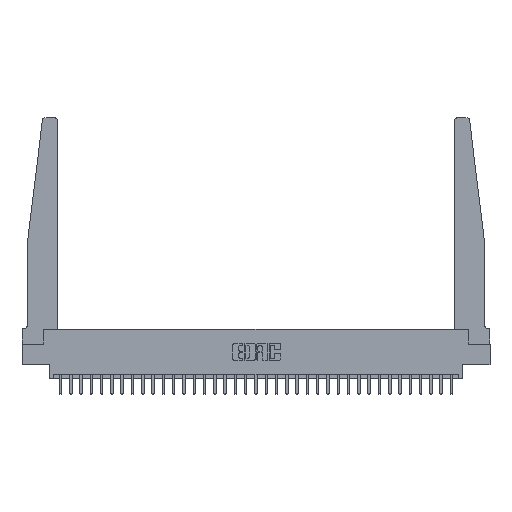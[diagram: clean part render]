
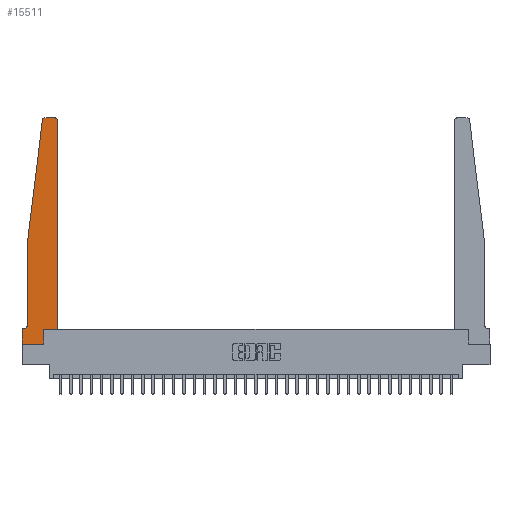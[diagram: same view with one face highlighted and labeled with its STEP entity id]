
A CAD part, top view. The second image highlights one B-rep face of the part: STEP entity #15511.
In plain terms, the highlighted planar face has unit normal (0, 0, 1).
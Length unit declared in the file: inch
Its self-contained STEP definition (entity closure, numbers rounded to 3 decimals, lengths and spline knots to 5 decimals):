
#685 = CARTESIAN_POINT ( 'NONE',  ( 0., 0.1875, 0.37 ) ) ;
#820 = VECTOR ( 'NONE', #7474, 39.37008 ) ;
#889 = ORIENTED_EDGE ( 'NONE', *, *, #24432, .T. ) ;
#991 = PLANE ( 'NONE',  #11258 ) ;
#1255 = CARTESIAN_POINT ( 'NONE',  ( 0.27653, 2.72, 0.37 ) ) ;
#1282 = CARTESIAN_POINT ( 'NONE',  ( 0.2605, 0.18, 0.37 ) ) ;
#1631 = CARTESIAN_POINT ( 'NONE',  ( 0.065, 1.25, 0.37 ) ) ;
#1986 = VECTOR ( 'NONE', #12154, 39.37008 ) ;
#2188 = DIRECTION ( 'NONE',  ( 0., 0., -1. ) ) ;
#2392 = LINE ( 'NONE', #28717, #820 ) ;
#2483 = ORIENTED_EDGE ( 'NONE', *, *, #11545, .T. ) ;
#2834 = CIRCLE ( 'NONE', #11965, 0.03 ) ;
#3475 = VERTEX_POINT ( 'NONE', #19897 ) ;
#3646 = ORIENTED_EDGE ( 'NONE', *, *, #25849, .T. ) ;
#3796 = DIRECTION ( 'NONE',  ( 0., 0., 1. ) ) ;
#4072 = VERTEX_POINT ( 'NONE', #9542 ) ;
#4591 = VERTEX_POINT ( 'NONE', #9301 ) ;
#6393 = EDGE_CURVE ( 'NONE', #3475, #31056, #22093, .T. ) ;
#6551 = EDGE_CURVE ( 'NONE', #7473, #23028, #12603, .T. ) ;
#6651 = VECTOR ( 'NONE', #16238, 39.37008 ) ;
#6872 = EDGE_CURVE ( 'NONE', #4072, #24487, #2392, .T. ) ;
#6892 = VECTOR ( 'NONE', #14657, 39.37008 ) ;
#7473 = VERTEX_POINT ( 'NONE', #10303 ) ;
#7474 = DIRECTION ( 'NONE',  ( 1., 0., 0. ) ) ;
#7517 = CARTESIAN_POINT ( 'NONE',  ( 0., 0., 0.37 ) ) ;
#7569 = ORIENTED_EDGE ( 'NONE', *, *, #6872, .T. ) ;
#7737 = CARTESIAN_POINT ( 'NONE',  ( 0.425, 0.18, 0.37 ) ) ;
#7973 = DIRECTION ( 'NONE',  ( -1., 0., 0. ) ) ;
#7985 = EDGE_LOOP ( 'NONE', ( #17151, #16999, #26677, #23181, #26467, #3646, #2483, #27674, #29774, #7569, #28558, #889 ) ) ;
#8424 = CARTESIAN_POINT ( 'NONE',  ( 0.2605, 0., 0.37 ) ) ;
#8437 = CARTESIAN_POINT ( 'NONE',  ( 0.24675, 2.72367, 0.37 ) ) ;
#9171 = CARTESIAN_POINT ( 'NONE',  ( 0.395, 2.72, 0.37 ) ) ;
#9301 = CARTESIAN_POINT ( 'NONE',  ( 0., 0.1875, 0.37 ) ) ;
#9408 = VERTEX_POINT ( 'NONE', #25878 ) ;
#9542 = CARTESIAN_POINT ( 'NONE',  ( 0.2605, 0.18, 0.37 ) ) ;
#10295 = VECTOR ( 'NONE', #29173, 39.37008 ) ;
#10303 = CARTESIAN_POINT ( 'NONE',  ( 0.395, 2.75, 0.37 ) ) ;
#10455 = EDGE_CURVE ( 'NONE', #24487, #24662, #17054, .T. ) ;
#10781 = DIRECTION ( 'NONE',  ( 0., -1., 0. ) ) ;
#11258 = AXIS2_PLACEMENT_3D ( 'NONE', #685, #12611, #24957 ) ;
#11545 = EDGE_CURVE ( 'NONE', #4591, #3475, #15531, .T. ) ;
#11681 = CARTESIAN_POINT ( 'NONE',  ( 0.27653, 2.75, 0.37 ) ) ;
#11965 = AXIS2_PLACEMENT_3D ( 'NONE', #9171, #23437, #14410 ) ;
#12154 = DIRECTION ( 'NONE',  ( 0., 1., 0. ) ) ;
#12603 = LINE ( 'NONE', #27469, #29700 ) ;
#12611 = DIRECTION ( 'NONE',  ( 0., 0., 1. ) ) ;
#12852 = EDGE_CURVE ( 'NONE', #16653, #12929, #13551, .T. ) ;
#12929 = VERTEX_POINT ( 'NONE', #19401 ) ;
#13484 = DIRECTION ( 'NONE',  ( 1., 0., 0. ) ) ;
#13551 = LINE ( 'NONE', #1631, #6651 ) ;
#13776 = DIRECTION ( 'NONE',  ( -1., 0., 0. ) ) ;
#14043 = AXIS2_PLACEMENT_3D ( 'NONE', #28671, #2188, #13776 ) ;
#14125 = LINE ( 'NONE', #16349, #21555 ) ;
#14410 = DIRECTION ( 'NONE',  ( 1., 0., 0. ) ) ;
#14657 = DIRECTION ( 'NONE',  ( 1., 0., 0. ) ) ;
#15228 = VECTOR ( 'NONE', #10781, 39.37008 ) ;
#15511 = ADVANCED_FACE ( 'NONE', ( #27172 ), #991, .T. ) ;
#15531 = LINE ( 'NONE', #25192, #15228 ) ;
#16076 = CARTESIAN_POINT ( 'NONE',  ( 0.425, 2.72, 0.37 ) ) ;
#16192 = EDGE_CURVE ( 'NONE', #23028, #18511, #17373, .T. ) ;
#16238 = DIRECTION ( 'NONE',  ( 0., -1., 0. ) ) ;
#16349 = CARTESIAN_POINT ( 'NONE',  ( 0.065, 0.1875, 0.37 ) ) ;
#16653 = VERTEX_POINT ( 'NONE', #19744 ) ;
#16999 = ORIENTED_EDGE ( 'NONE', *, *, #16192, .T. ) ;
#17054 = LINE ( 'NONE', #24657, #1986 ) ;
#17151 = ORIENTED_EDGE ( 'NONE', *, *, #6551, .T. ) ;
#17373 = CIRCLE ( 'NONE', #18875, 0.03 ) ;
#18511 = VERTEX_POINT ( 'NONE', #8437 ) ;
#18875 = AXIS2_PLACEMENT_3D ( 'NONE', #1255, #3796, #13484 ) ;
#19019 = CARTESIAN_POINT ( 'NONE',  ( 0.065, 1.25, 0.37 ) ) ;
#19401 = CARTESIAN_POINT ( 'NONE',  ( 0.065, 0.2375, 0.37 ) ) ;
#19744 = CARTESIAN_POINT ( 'NONE',  ( 0.065, 1.25, 0.37 ) ) ;
#19897 = CARTESIAN_POINT ( 'NONE',  ( 0., 0., 0.37 ) ) ;
#20652 = EDGE_CURVE ( 'NONE', #18511, #16653, #21394, .T. ) ;
#21394 = LINE ( 'NONE', #19019, #10295 ) ;
#21555 = VECTOR ( 'NONE', #26008, 39.37008 ) ;
#22093 = LINE ( 'NONE', #7517, #6892 ) ;
#23028 = VERTEX_POINT ( 'NONE', #11681 ) ;
#23181 = ORIENTED_EDGE ( 'NONE', *, *, #12852, .T. ) ;
#23437 = DIRECTION ( 'NONE',  ( 0., 0., 1. ) ) ;
#24432 = EDGE_CURVE ( 'NONE', #24662, #7473, #2834, .T. ) ;
#24487 = VERTEX_POINT ( 'NONE', #7737 ) ;
#24657 = CARTESIAN_POINT ( 'NONE',  ( 0.425, 0.18, 0.37 ) ) ;
#24662 = VERTEX_POINT ( 'NONE', #16076 ) ;
#24957 = DIRECTION ( 'NONE',  ( 1., 0., 0. ) ) ;
#25176 = CIRCLE ( 'NONE', #14043, 0.05 ) ;
#25192 = CARTESIAN_POINT ( 'NONE',  ( 0., 0., 0.37 ) ) ;
#25245 = LINE ( 'NONE', #1282, #29217 ) ;
#25704 = DIRECTION ( 'NONE',  ( 0., 1., 0. ) ) ;
#25849 = EDGE_CURVE ( 'NONE', #9408, #4591, #14125, .T. ) ;
#25878 = CARTESIAN_POINT ( 'NONE',  ( 0.015, 0.1875, 0.37 ) ) ;
#26008 = DIRECTION ( 'NONE',  ( -1., 0., 0. ) ) ;
#26467 = ORIENTED_EDGE ( 'NONE', *, *, #27577, .T. ) ;
#26677 = ORIENTED_EDGE ( 'NONE', *, *, #20652, .T. ) ;
#26973 = EDGE_CURVE ( 'NONE', #31056, #4072, #25245, .T. ) ;
#27172 = FACE_OUTER_BOUND ( 'NONE', #7985, .T. ) ;
#27469 = CARTESIAN_POINT ( 'NONE',  ( 0.25, 2.75, 0.37 ) ) ;
#27577 = EDGE_CURVE ( 'NONE', #12929, #9408, #25176, .T. ) ;
#27674 = ORIENTED_EDGE ( 'NONE', *, *, #6393, .T. ) ;
#28558 = ORIENTED_EDGE ( 'NONE', *, *, #10455, .T. ) ;
#28671 = CARTESIAN_POINT ( 'NONE',  ( 0.015, 0.2375, 0.37 ) ) ;
#28717 = CARTESIAN_POINT ( 'NONE',  ( 0.425, 0.18, 0.37 ) ) ;
#29173 = DIRECTION ( 'NONE',  ( -0.122, -0.992, 0. ) ) ;
#29217 = VECTOR ( 'NONE', #25704, 39.37008 ) ;
#29700 = VECTOR ( 'NONE', #7973, 39.37008 ) ;
#29774 = ORIENTED_EDGE ( 'NONE', *, *, #26973, .T. ) ;
#31056 = VERTEX_POINT ( 'NONE', #8424 ) ;
